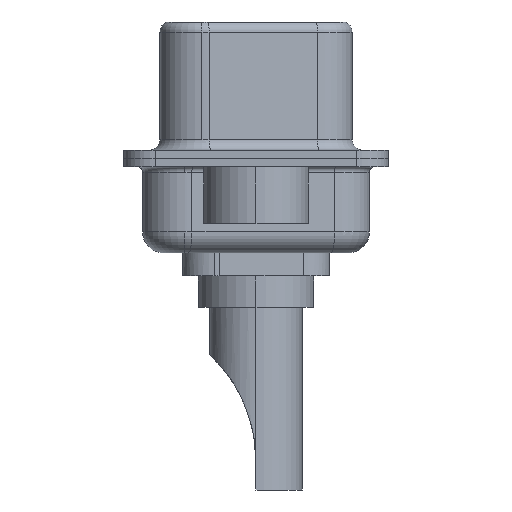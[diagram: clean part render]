
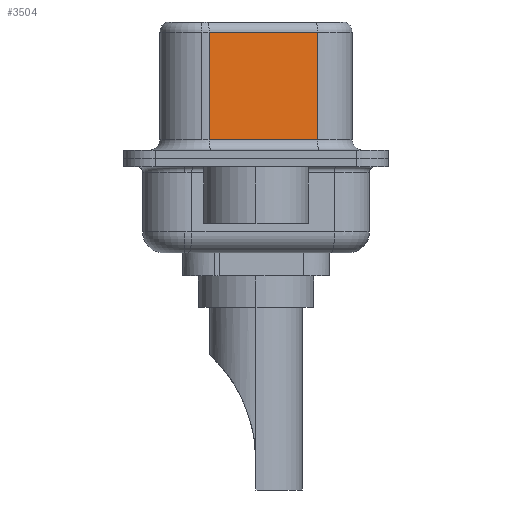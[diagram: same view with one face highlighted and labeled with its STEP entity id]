
A CAD part, left-side view. The second image highlights one B-rep face of the part: STEP entity #3504.
In plain terms, the highlighted planar face has unit normal (-0.985, -0.174, 0).
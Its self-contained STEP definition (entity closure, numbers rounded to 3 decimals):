
#517 = EDGE_CURVE ( 'NONE', #1486, #898, #12773, .T. ) ;
#875 = CARTESIAN_POINT ( 'NONE',  ( 4.565, -2.927, 6.52 ) ) ;
#898 = VERTEX_POINT ( 'NONE', #2073 ) ;
#1486 = VERTEX_POINT ( 'NONE', #13501 ) ;
#1553 = VECTOR ( 'NONE', #8246, 1000. ) ;
#2073 = CARTESIAN_POINT ( 'NONE',  ( 4.565, -2.927, 0.9 ) ) ;
#2080 = FACE_OUTER_BOUND ( 'NONE', #8546, .T. ) ;
#3018 = VERTEX_POINT ( 'NONE', #12670 ) ;
#3431 = DIRECTION ( 'NONE',  ( 0.174, -0.985, 0. ) ) ;
#3504 = ADVANCED_FACE ( 'NONE', ( #2080 ), #11451, .F. ) ;
#3845 = DIRECTION ( 'NONE',  ( -0.174, 0.985, 0. ) ) ;
#4675 = ORIENTED_EDGE ( 'NONE', *, *, #14981, .T. ) ;
#5185 = LINE ( 'NONE', #5589, #14288 ) ;
#5589 = CARTESIAN_POINT ( 'NONE',  ( 3.655, 2.233, 6.52 ) ) ;
#6090 = ORIENTED_EDGE ( 'NONE', *, *, #14671, .T. ) ;
#6680 = CARTESIAN_POINT ( 'NONE',  ( 4.565, -2.927, 0.9 ) ) ;
#7497 = LINE ( 'NONE', #14964, #14084 ) ;
#8246 = DIRECTION ( 'NONE',  ( 0., 0., -1. ) ) ;
#8546 = EDGE_LOOP ( 'NONE', ( #10615, #4675, #6090, #11663 ) ) ;
#9136 = VECTOR ( 'NONE', #3431, 1000. ) ;
#9146 = AXIS2_PLACEMENT_3D ( 'NONE', #10945, #10791, #10613 ) ;
#9372 = CARTESIAN_POINT ( 'NONE',  ( 3.655, 2.233, 6.02 ) ) ;
#10613 = DIRECTION ( 'NONE',  ( -0.174, 0.985, 0. ) ) ;
#10615 = ORIENTED_EDGE ( 'NONE', *, *, #11946, .F. ) ;
#10791 = DIRECTION ( 'NONE',  ( 0.985, 0.174, 0. ) ) ;
#10945 = CARTESIAN_POINT ( 'NONE',  ( 4.565, -2.927, 6.52 ) ) ;
#10985 = LINE ( 'NONE', #875, #1553 ) ;
#11451 = PLANE ( 'NONE',  #9146 ) ;
#11663 = ORIENTED_EDGE ( 'NONE', *, *, #517, .T. ) ;
#11946 = EDGE_CURVE ( 'NONE', #3018, #898, #10985, .T. ) ;
#12670 = CARTESIAN_POINT ( 'NONE',  ( 4.565, -2.927, 6.02 ) ) ;
#12773 = LINE ( 'NONE', #6680, #9136 ) ;
#13501 = CARTESIAN_POINT ( 'NONE',  ( 3.655, 2.233, 0.9 ) ) ;
#14084 = VECTOR ( 'NONE', #3845, 1000. ) ;
#14264 = DIRECTION ( 'NONE',  ( 0., 0., -1. ) ) ;
#14288 = VECTOR ( 'NONE', #14264, 1000. ) ;
#14671 = EDGE_CURVE ( 'NONE', #15369, #1486, #5185, .T. ) ;
#14964 = CARTESIAN_POINT ( 'NONE',  ( 4.565, -2.927, 6.02 ) ) ;
#14981 = EDGE_CURVE ( 'NONE', #3018, #15369, #7497, .T. ) ;
#15369 = VERTEX_POINT ( 'NONE', #9372 ) ;
